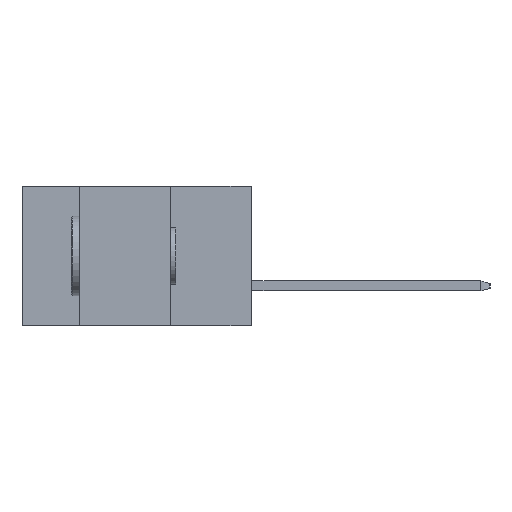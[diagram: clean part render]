
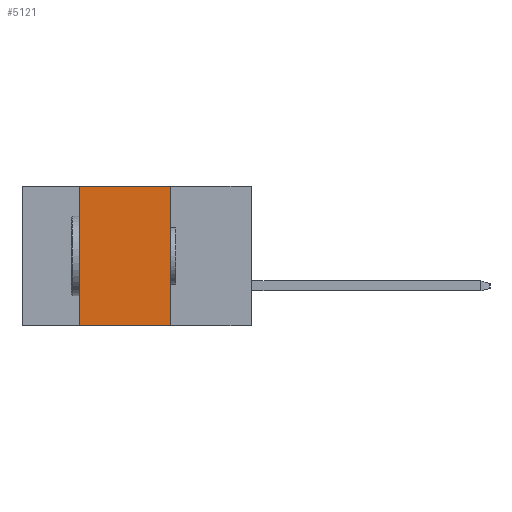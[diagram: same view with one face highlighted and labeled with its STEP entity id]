
A CAD part, left-side view. The second image highlights one B-rep face of the part: STEP entity #5121.
In plain terms, the highlighted planar face has unit normal (-1, 0, 0).
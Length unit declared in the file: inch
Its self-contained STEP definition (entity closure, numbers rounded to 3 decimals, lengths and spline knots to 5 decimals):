
#326 = AXIS2_PLACEMENT_3D ( 'NONE', #2133, #583, #9295 ) ;
#583 = DIRECTION ( 'NONE',  ( 1., 0., 0. ) ) ;
#766 = CARTESIAN_POINT ( 'NONE',  ( 0., 0.72, 0. ) ) ;
#1436 = ORIENTED_EDGE ( 'NONE', *, *, #4745, .T. ) ;
#1908 = EDGE_LOOP ( 'NONE', ( #7341, #3706, #2287, #1436 ) ) ;
#2133 = CARTESIAN_POINT ( 'NONE',  ( 0., 0.72, 0. ) ) ;
#2146 = CARTESIAN_POINT ( 'NONE',  ( 0., 0.72, -0.437 ) ) ;
#2287 = ORIENTED_EDGE ( 'NONE', *, *, #9874, .F. ) ;
#2740 = VERTEX_POINT ( 'NONE', #7366 ) ;
#2925 = LINE ( 'NONE', #2146, #2974 ) ;
#2951 = VERTEX_POINT ( 'NONE', #8547 ) ;
#2960 = EDGE_CURVE ( 'NONE', #6992, #4487, #2991, .T. ) ;
#2974 = VECTOR ( 'NONE', #5325, 39.37008 ) ;
#2991 = LINE ( 'NONE', #8395, #9732 ) ;
#3706 = ORIENTED_EDGE ( 'NONE', *, *, #7297, .F. ) ;
#4487 = VERTEX_POINT ( 'NONE', #9009 ) ;
#4682 = CARTESIAN_POINT ( 'NONE',  ( 0., 0.254, 0. ) ) ;
#4709 = LINE ( 'NONE', #766, #9108 ) ;
#4745 = EDGE_CURVE ( 'NONE', #2951, #4487, #2925, .T. ) ;
#5121 = ADVANCED_FACE ( 'NONE', ( #7595 ), #9246, .F. ) ;
#5251 = DIRECTION ( 'NONE',  ( 0., -1., 0. ) ) ;
#5325 = DIRECTION ( 'NONE',  ( 0., -1., 0. ) ) ;
#5428 = DIRECTION ( 'NONE',  ( 0., 0., -1. ) ) ;
#6992 = VERTEX_POINT ( 'NONE', #4682 ) ;
#7065 = DIRECTION ( 'NONE',  ( 0., 0., 1. ) ) ;
#7297 = EDGE_CURVE ( 'NONE', #2740, #6992, #4709, .T. ) ;
#7341 = ORIENTED_EDGE ( 'NONE', *, *, #2960, .F. ) ;
#7366 = CARTESIAN_POINT ( 'NONE',  ( 0., 0.54, 0. ) ) ;
#7595 = FACE_OUTER_BOUND ( 'NONE', #1908, .T. ) ;
#7896 = CARTESIAN_POINT ( 'NONE',  ( 0., 0.54, -0.437 ) ) ;
#8395 = CARTESIAN_POINT ( 'NONE',  ( 0., 0.254, -0.437 ) ) ;
#8547 = CARTESIAN_POINT ( 'NONE',  ( 0., 0.54, -0.437 ) ) ;
#9009 = CARTESIAN_POINT ( 'NONE',  ( 0., 0.254, -0.437 ) ) ;
#9108 = VECTOR ( 'NONE', #5251, 39.37008 ) ;
#9246 = PLANE ( 'NONE',  #326 ) ;
#9295 = DIRECTION ( 'NONE',  ( 0., 0., -1. ) ) ;
#9488 = LINE ( 'NONE', #7896, #9504 ) ;
#9504 = VECTOR ( 'NONE', #7065, 39.37008 ) ;
#9732 = VECTOR ( 'NONE', #5428, 39.37008 ) ;
#9874 = EDGE_CURVE ( 'NONE', #2951, #2740, #9488, .T. ) ;
